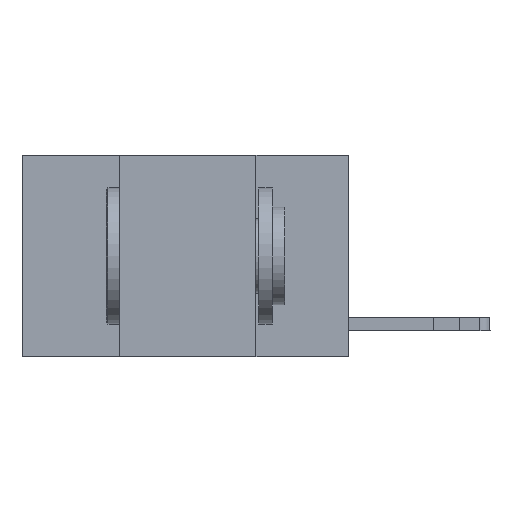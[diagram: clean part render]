
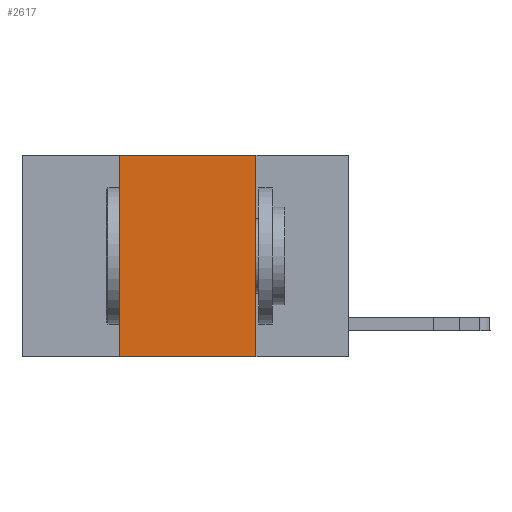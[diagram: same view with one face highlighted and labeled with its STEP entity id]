
A CAD part, left-side view. The second image highlights one B-rep face of the part: STEP entity #2617.
In plain terms, the highlighted planar face has unit normal (-1, 0, 0).
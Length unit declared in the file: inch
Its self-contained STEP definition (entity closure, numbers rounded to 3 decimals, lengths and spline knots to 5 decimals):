
#281 = ORIENTED_EDGE ( 'NONE', *, *, #3345, .F. ) ;
#871 = ORIENTED_EDGE ( 'NONE', *, *, #7126, .T. ) ;
#915 = DIRECTION ( 'NONE',  ( 0., 0., -1. ) ) ;
#921 = LINE ( 'NONE', #7968, #8751 ) ;
#1018 = DIRECTION ( 'NONE',  ( 0., -1., 0. ) ) ;
#1441 = CARTESIAN_POINT ( 'NONE',  ( 0., 0.42, 0. ) ) ;
#2504 = DIRECTION ( 'NONE',  ( 0., 0., -1. ) ) ;
#2617 = ADVANCED_FACE ( 'NONE', ( #9906 ), #10207, .F. ) ;
#3075 = DIRECTION ( 'NONE',  ( 0., -1., 0. ) ) ;
#3087 = CARTESIAN_POINT ( 'NONE',  ( 0., 0.42, 0. ) ) ;
#3345 = EDGE_CURVE ( 'NONE', #9814, #12057, #4680, .T. ) ;
#3543 = CARTESIAN_POINT ( 'NONE',  ( 0., 0.6, 0. ) ) ;
#4196 = LINE ( 'NONE', #3087, #6560 ) ;
#4366 = CARTESIAN_POINT ( 'NONE',  ( 0., 0.17, -0.37 ) ) ;
#4411 = EDGE_CURVE ( 'NONE', #5789, #9022, #4196, .T. ) ;
#4680 = LINE ( 'NONE', #5757, #10577 ) ;
#4910 = LINE ( 'NONE', #7101, #5689 ) ;
#5689 = VECTOR ( 'NONE', #1018, 39.37008 ) ;
#5757 = CARTESIAN_POINT ( 'NONE',  ( 0., 0.17, 0. ) ) ;
#5789 = VERTEX_POINT ( 'NONE', #11381 ) ;
#6297 = DIRECTION ( 'NONE',  ( 1., 0., 0. ) ) ;
#6560 = VECTOR ( 'NONE', #8037, 39.37008 ) ;
#7101 = CARTESIAN_POINT ( 'NONE',  ( 0., 0.6, -0.37 ) ) ;
#7126 = EDGE_CURVE ( 'NONE', #5789, #12057, #4910, .T. ) ;
#7968 = CARTESIAN_POINT ( 'NONE',  ( 0., 0.6, 0. ) ) ;
#8037 = DIRECTION ( 'NONE',  ( 0., 0., 1. ) ) ;
#8552 = EDGE_CURVE ( 'NONE', #9022, #9814, #921, .T. ) ;
#8751 = VECTOR ( 'NONE', #3075, 39.37008 ) ;
#8804 = ORIENTED_EDGE ( 'NONE', *, *, #8552, .F. ) ;
#9022 = VERTEX_POINT ( 'NONE', #1441 ) ;
#9156 = CARTESIAN_POINT ( 'NONE',  ( 0., 0.17, 0. ) ) ;
#9712 = ORIENTED_EDGE ( 'NONE', *, *, #4411, .F. ) ;
#9814 = VERTEX_POINT ( 'NONE', #9156 ) ;
#9906 = FACE_OUTER_BOUND ( 'NONE', #10265, .T. ) ;
#10207 = PLANE ( 'NONE',  #11977 ) ;
#10265 = EDGE_LOOP ( 'NONE', ( #281, #8804, #9712, #871 ) ) ;
#10577 = VECTOR ( 'NONE', #915, 39.37008 ) ;
#11381 = CARTESIAN_POINT ( 'NONE',  ( 0., 0.42, -0.37 ) ) ;
#11977 = AXIS2_PLACEMENT_3D ( 'NONE', #3543, #6297, #2504 ) ;
#12057 = VERTEX_POINT ( 'NONE', #4366 ) ;
